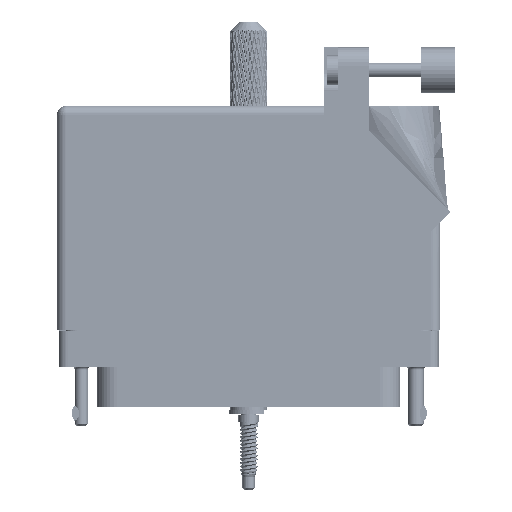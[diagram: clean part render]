
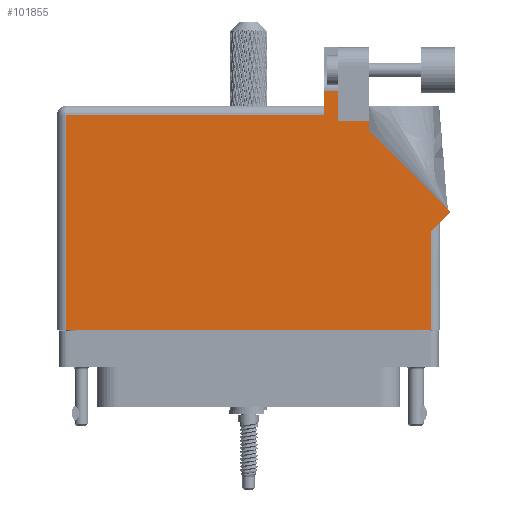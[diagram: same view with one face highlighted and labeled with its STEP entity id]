
A CAD part, front view. The second image highlights one B-rep face of the part: STEP entity #101855.
In plain terms, the highlighted face is planar.
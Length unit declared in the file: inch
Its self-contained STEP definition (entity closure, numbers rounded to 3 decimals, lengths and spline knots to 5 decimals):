
#360 = DIRECTION ( 'NONE',  ( -1., 0., 0. ) ) ;
#803 = CARTESIAN_POINT ( 'NONE',  ( 0.82, 1.26442, 0.455 ) ) ;
#1626 = LINE ( 'NONE', #70472, #85655 ) ;
#7125 = LINE ( 'NONE', #25136, #71730 ) ;
#7849 = EDGE_LOOP ( 'NONE', ( #38458, #70666, #91172, #29100, #51307, #105768, #77265, #75138, #14367, #56132, #84323 ) ) ;
#10064 = CARTESIAN_POINT ( 'NONE',  ( 0.82, 1.26442, 0.455 ) ) ;
#10114 = CARTESIAN_POINT ( 'NONE',  ( 0.607, 1.5315, 0.455 ) ) ;
#10541 = CARTESIAN_POINT ( 'NONE',  ( -1.306, 1.368, 0.455 ) ) ;
#10974 = DIRECTION ( 'NONE',  ( 0., -1., 0. ) ) ;
#11043 = CARTESIAN_POINT ( 'NONE',  ( 0.513, 1.5315, 0.455 ) ) ;
#13044 = CARTESIAN_POINT ( 'NONE',  ( 1.37671, 0.70771, 0.455 ) ) ;
#13233 = LINE ( 'NONE', #33157, #87036 ) ;
#13688 = DIRECTION ( 'NONE',  ( -0.707, 0.707, 0. ) ) ;
#14367 = ORIENTED_EDGE ( 'NONE', *, *, #116149, .T. ) ;
#15509 = DIRECTION ( 'NONE',  ( 1., 0., 0. ) ) ;
#17498 = CARTESIAN_POINT ( 'NONE',  ( -1.244, 1.368, 0.455 ) ) ;
#18890 = CARTESIAN_POINT ( 'NONE',  ( 0.607, 1.33, 0.455 ) ) ;
#20835 = LINE ( 'NONE', #10541, #125967 ) ;
#25136 = CARTESIAN_POINT ( 'NONE',  ( -1.306, -0.1, 0.455 ) ) ;
#25507 = VECTOR ( 'NONE', #111567, 39.37008 ) ;
#25890 = VECTOR ( 'NONE', #45530, 39.37008 ) ;
#29100 = ORIENTED_EDGE ( 'NONE', *, *, #61063, .T. ) ;
#30339 = LINE ( 'NONE', #64367, #41641 ) ;
#30693 = EDGE_CURVE ( 'NONE', #49291, #124737, #88874, .T. ) ;
#31839 = CARTESIAN_POINT ( 'NONE',  ( -1.306, 1.43, 0.455 ) ) ;
#31991 = VERTEX_POINT ( 'NONE', #97126 ) ;
#33109 = DIRECTION ( 'NONE',  ( -1., 0., 0. ) ) ;
#33157 = CARTESIAN_POINT ( 'NONE',  ( -1.244, -0.1, 0.455 ) ) ;
#33769 = CARTESIAN_POINT ( 'NONE',  ( 0.513, 1.368, 0.455 ) ) ;
#36238 = CARTESIAN_POINT ( 'NONE',  ( 1.37671, 0.70771, 0.455 ) ) ;
#38458 = ORIENTED_EDGE ( 'NONE', *, *, #72816, .T. ) ;
#41641 = VECTOR ( 'NONE', #73416, 39.37008 ) ;
#42137 = PLANE ( 'NONE',  #57158 ) ;
#42672 = VERTEX_POINT ( 'NONE', #119878 ) ;
#44046 = EDGE_CURVE ( 'NONE', #55141, #49291, #1626, .T. ) ;
#45530 = DIRECTION ( 'NONE',  ( -1., 0., 0. ) ) ;
#46820 = CARTESIAN_POINT ( 'NONE',  ( 0.82, 1.33, 0.455 ) ) ;
#47942 = VERTEX_POINT ( 'NONE', #10064 ) ;
#49291 = VERTEX_POINT ( 'NONE', #11043 ) ;
#51307 = ORIENTED_EDGE ( 'NONE', *, *, #70421, .T. ) ;
#55141 = VERTEX_POINT ( 'NONE', #10114 ) ;
#56132 = ORIENTED_EDGE ( 'NONE', *, *, #100252, .T. ) ;
#57158 = AXIS2_PLACEMENT_3D ( 'NONE', #31839, #100083, #33109 ) ;
#61063 = EDGE_CURVE ( 'NONE', #124737, #113808, #20835, .T. ) ;
#62073 = FACE_OUTER_BOUND ( 'NONE', #7849, .T. ) ;
#64355 = VECTOR ( 'NONE', #13688, 39.37008 ) ;
#64367 = CARTESIAN_POINT ( 'NONE',  ( 1.244, 0.637, 0.455 ) ) ;
#64433 = CARTESIAN_POINT ( 'NONE',  ( 1.244, 0.575, 0.455 ) ) ;
#70362 = DIRECTION ( 'NONE',  ( -1., 0., 0. ) ) ;
#70421 = EDGE_CURVE ( 'NONE', #113808, #42672, #13233, .T. ) ;
#70472 = CARTESIAN_POINT ( 'NONE',  ( 0.93777, 1.5315, 0.455 ) ) ;
#70666 = ORIENTED_EDGE ( 'NONE', *, *, #44046, .T. ) ;
#71058 = CARTESIAN_POINT ( 'NONE',  ( 0.607, 1.33, 0.455 ) ) ;
#71730 = VECTOR ( 'NONE', #15509, 39.37008 ) ;
#72816 = EDGE_CURVE ( 'NONE', #96034, #55141, #82010, .T. ) ;
#73416 = DIRECTION ( 'NONE',  ( 0., 1., 0. ) ) ;
#75138 = ORIENTED_EDGE ( 'NONE', *, *, #111277, .T. ) ;
#77265 = ORIENTED_EDGE ( 'NONE', *, *, #115664, .T. ) ;
#79564 = VECTOR ( 'NONE', #90250, 39.37008 ) ;
#82010 = LINE ( 'NONE', #71058, #25507 ) ;
#84323 = ORIENTED_EDGE ( 'NONE', *, *, #98101, .T. ) ;
#85655 = VECTOR ( 'NONE', #360, 39.37008 ) ;
#86108 = VERTEX_POINT ( 'NONE', #36238 ) ;
#87036 = VECTOR ( 'NONE', #100750, 39.37008 ) ;
#88799 = CARTESIAN_POINT ( 'NONE',  ( 1.244, -0.1, 0.455 ) ) ;
#88874 = LINE ( 'NONE', #90767, #119942 ) ;
#88979 = LINE ( 'NONE', #803, #79564 ) ;
#90250 = DIRECTION ( 'NONE',  ( 0., 1., 0. ) ) ;
#90767 = CARTESIAN_POINT ( 'NONE',  ( 0.513, 1.43, 0.455 ) ) ;
#91172 = ORIENTED_EDGE ( 'NONE', *, *, #30693, .T. ) ;
#92880 = CARTESIAN_POINT ( 'NONE',  ( 1.306, 0.637, 0.455 ) ) ;
#96034 = VERTEX_POINT ( 'NONE', #18890 ) ;
#97126 = CARTESIAN_POINT ( 'NONE',  ( 0.82, 1.33, 0.455 ) ) ;
#98101 = EDGE_CURVE ( 'NONE', #31991, #96034, #124027, .T. ) ;
#100083 = DIRECTION ( 'NONE',  ( 0., 0., -1. ) ) ;
#100252 = EDGE_CURVE ( 'NONE', #47942, #31991, #88979, .T. ) ;
#100750 = DIRECTION ( 'NONE',  ( 0., -1., 0. ) ) ;
#101216 = VERTEX_POINT ( 'NONE', #64433 ) ;
#101855 = ADVANCED_FACE ( 'NONE', ( #62073 ), #42137, .F. ) ;
#103159 = LINE ( 'NONE', #92880, #109119 ) ;
#105768 = ORIENTED_EDGE ( 'NONE', *, *, #120116, .T. ) ;
#107673 = VERTEX_POINT ( 'NONE', #88799 ) ;
#109119 = VECTOR ( 'NONE', #112188, 39.37008 ) ;
#111277 = EDGE_CURVE ( 'NONE', #101216, #86108, #103159, .T. ) ;
#111567 = DIRECTION ( 'NONE',  ( 0., 1., 0. ) ) ;
#112188 = DIRECTION ( 'NONE',  ( 0.707, 0.707, 0. ) ) ;
#113808 = VERTEX_POINT ( 'NONE', #17498 ) ;
#115664 = EDGE_CURVE ( 'NONE', #107673, #101216, #30339, .T. ) ;
#116149 = EDGE_CURVE ( 'NONE', #86108, #47942, #121138, .T. ) ;
#119878 = CARTESIAN_POINT ( 'NONE',  ( -1.244, -0.1, 0.455 ) ) ;
#119942 = VECTOR ( 'NONE', #10974, 39.37008 ) ;
#120116 = EDGE_CURVE ( 'NONE', #42672, #107673, #7125, .T. ) ;
#121138 = LINE ( 'NONE', #13044, #64355 ) ;
#124027 = LINE ( 'NONE', #46820, #25890 ) ;
#124737 = VERTEX_POINT ( 'NONE', #33769 ) ;
#125967 = VECTOR ( 'NONE', #70362, 39.37008 ) ;
